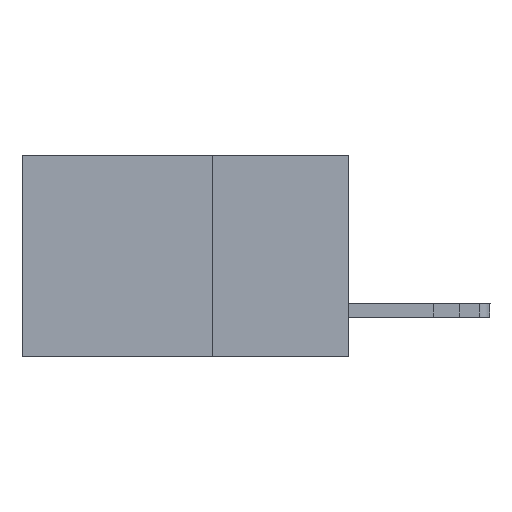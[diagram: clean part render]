
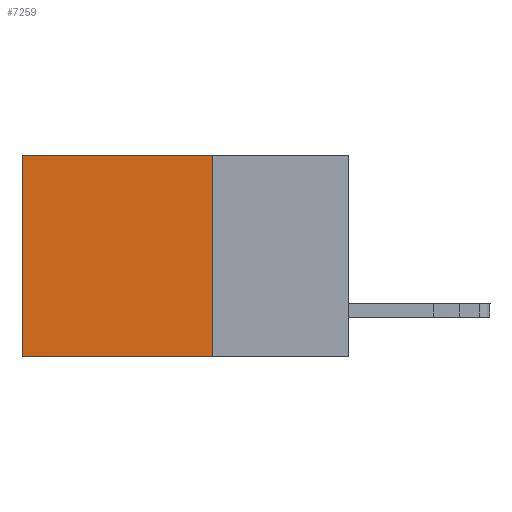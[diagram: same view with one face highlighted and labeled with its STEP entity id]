
A CAD part, left-side view. The second image highlights one B-rep face of the part: STEP entity #7259.
In plain terms, the highlighted planar face has unit normal (-1, 0, 0).
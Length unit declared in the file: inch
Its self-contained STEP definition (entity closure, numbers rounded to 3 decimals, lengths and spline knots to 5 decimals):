
#116 = CARTESIAN_POINT ( 'NONE',  ( 0.2615, 0.25, -0.37 ) ) ;
#774 = CARTESIAN_POINT ( 'NONE',  ( 0.2615, 0.25, -0.37 ) ) ;
#924 = ORIENTED_EDGE ( 'NONE', *, *, #11495, .T. ) ;
#1102 = CARTESIAN_POINT ( 'NONE',  ( 0.2615, 0.6, -0.37 ) ) ;
#1117 = DIRECTION ( 'NONE',  ( 0., 0., -1. ) ) ;
#1339 = CARTESIAN_POINT ( 'NONE',  ( 0.2615, 0.25, 0. ) ) ;
#1367 = CARTESIAN_POINT ( 'NONE',  ( 0.2615, 0.25, -0.37 ) ) ;
#1815 = LINE ( 'NONE', #8173, #12419 ) ;
#1842 = DIRECTION ( 'NONE',  ( 0., 1., 0. ) ) ;
#2136 = VERTEX_POINT ( 'NONE', #1339 ) ;
#2322 = DIRECTION ( 'NONE',  ( 0., 0., -1. ) ) ;
#2808 = VECTOR ( 'NONE', #7509, 39.37008 ) ;
#3049 = ORIENTED_EDGE ( 'NONE', *, *, #5232, .F. ) ;
#3214 = ORIENTED_EDGE ( 'NONE', *, *, #6758, .T. ) ;
#4465 = VERTEX_POINT ( 'NONE', #11359 ) ;
#5232 = EDGE_CURVE ( 'NONE', #2136, #11316, #8893, .T. ) ;
#5434 = LINE ( 'NONE', #10337, #2808 ) ;
#6031 = VERTEX_POINT ( 'NONE', #1102 ) ;
#6076 = PLANE ( 'NONE',  #8923 ) ;
#6433 = FACE_OUTER_BOUND ( 'NONE', #11742, .T. ) ;
#6530 = LINE ( 'NONE', #7726, #9078 ) ;
#6758 = EDGE_CURVE ( 'NONE', #4465, #6031, #1815, .T. ) ;
#7054 = DIRECTION ( 'NONE',  ( 1., 0., 0. ) ) ;
#7259 = ADVANCED_FACE ( 'NONE', ( #6433 ), #6076, .F. ) ;
#7509 = DIRECTION ( 'NONE',  ( 0., 1., 0. ) ) ;
#7726 = CARTESIAN_POINT ( 'NONE',  ( 0.2615, 0.25, -0.37 ) ) ;
#8173 = CARTESIAN_POINT ( 'NONE',  ( 0.2615, 0.6, -0.37 ) ) ;
#8893 = LINE ( 'NONE', #774, #11140 ) ;
#8923 = AXIS2_PLACEMENT_3D ( 'NONE', #116, #7054, #1117 ) ;
#9078 = VECTOR ( 'NONE', #1842, 39.37008 ) ;
#9810 = ORIENTED_EDGE ( 'NONE', *, *, #11623, .F. ) ;
#10337 = CARTESIAN_POINT ( 'NONE',  ( 0.2615, 0.25, 0. ) ) ;
#11140 = VECTOR ( 'NONE', #12413, 39.37008 ) ;
#11316 = VERTEX_POINT ( 'NONE', #1367 ) ;
#11359 = CARTESIAN_POINT ( 'NONE',  ( 0.2615, 0.6, 0. ) ) ;
#11495 = EDGE_CURVE ( 'NONE', #2136, #4465, #5434, .T. ) ;
#11623 = EDGE_CURVE ( 'NONE', #11316, #6031, #6530, .T. ) ;
#11742 = EDGE_LOOP ( 'NONE', ( #3214, #9810, #3049, #924 ) ) ;
#12413 = DIRECTION ( 'NONE',  ( 0., 0., -1. ) ) ;
#12419 = VECTOR ( 'NONE', #2322, 39.37008 ) ;
